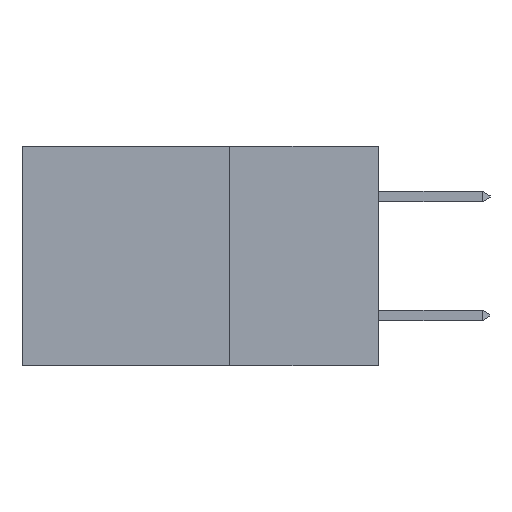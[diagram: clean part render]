
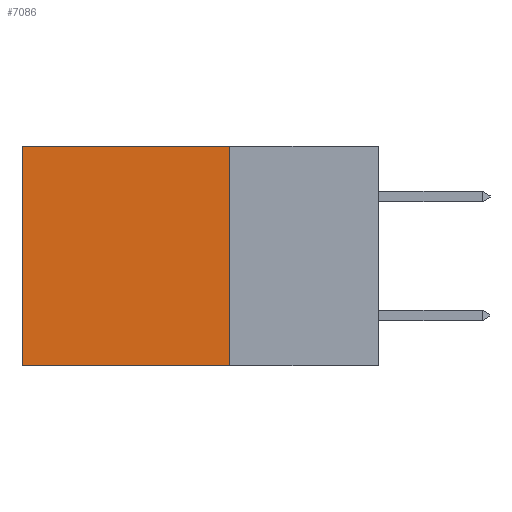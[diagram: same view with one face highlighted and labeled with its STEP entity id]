
A CAD part, left-side view. The second image highlights one B-rep face of the part: STEP entity #7086.
In plain terms, the highlighted planar face has unit normal (-1, 0, 0).
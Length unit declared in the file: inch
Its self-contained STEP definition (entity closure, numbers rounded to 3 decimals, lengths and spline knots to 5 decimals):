
#74 = CARTESIAN_POINT ( 'NONE',  ( 0.298, 0.6, 0. ) ) ;
#310 = EDGE_LOOP ( 'NONE', ( #7199, #5435, #2996, #6718 ) ) ;
#1851 = CARTESIAN_POINT ( 'NONE',  ( 0.298, 0.6, -0.37 ) ) ;
#2135 = LINE ( 'NONE', #3956, #12154 ) ;
#2180 = AXIS2_PLACEMENT_3D ( 'NONE', #2673, #4735, #11431 ) ;
#2197 = EDGE_CURVE ( 'NONE', #12668, #10796, #11174, .T. ) ;
#2673 = CARTESIAN_POINT ( 'NONE',  ( 0.298, 0.25, 0. ) ) ;
#2812 = CARTESIAN_POINT ( 'NONE',  ( 0.298, 0.25, 0. ) ) ;
#2899 = EDGE_CURVE ( 'NONE', #8520, #3314, #2135, .T. ) ;
#2996 = ORIENTED_EDGE ( 'NONE', *, *, #11598, .F. ) ;
#3002 = CARTESIAN_POINT ( 'NONE',  ( 0.298, 0.25, 0. ) ) ;
#3314 = VERTEX_POINT ( 'NONE', #74 ) ;
#3824 = DIRECTION ( 'NONE',  ( 0., 0., -1. ) ) ;
#3956 = CARTESIAN_POINT ( 'NONE',  ( 0.298, 0.25, 0. ) ) ;
#4020 = VECTOR ( 'NONE', #12395, 39.37008 ) ;
#4735 = DIRECTION ( 'NONE',  ( 1., 0., 0. ) ) ;
#5117 = LINE ( 'NONE', #2812, #10001 ) ;
#5435 = ORIENTED_EDGE ( 'NONE', *, *, #2197, .F. ) ;
#5853 = CARTESIAN_POINT ( 'NONE',  ( 0.298, 0.25, -0.37 ) ) ;
#6718 = ORIENTED_EDGE ( 'NONE', *, *, #2899, .T. ) ;
#7034 = CARTESIAN_POINT ( 'NONE',  ( 0.298, 0.25, -0.37 ) ) ;
#7086 = ADVANCED_FACE ( 'NONE', ( #9249 ), #10544, .F. ) ;
#7199 = ORIENTED_EDGE ( 'NONE', *, *, #8305, .T. ) ;
#8305 = EDGE_CURVE ( 'NONE', #3314, #10796, #11991, .T. ) ;
#8520 = VERTEX_POINT ( 'NONE', #3002 ) ;
#8833 = VECTOR ( 'NONE', #12445, 39.37008 ) ;
#9249 = FACE_OUTER_BOUND ( 'NONE', #310, .T. ) ;
#10001 = VECTOR ( 'NONE', #3824, 39.37008 ) ;
#10341 = DIRECTION ( 'NONE',  ( 0., 1., 0. ) ) ;
#10544 = PLANE ( 'NONE',  #2180 ) ;
#10796 = VERTEX_POINT ( 'NONE', #1851 ) ;
#11174 = LINE ( 'NONE', #5853, #8833 ) ;
#11431 = DIRECTION ( 'NONE',  ( 0., 0., -1. ) ) ;
#11495 = CARTESIAN_POINT ( 'NONE',  ( 0.298, 0.6, 0. ) ) ;
#11598 = EDGE_CURVE ( 'NONE', #8520, #12668, #5117, .T. ) ;
#11991 = LINE ( 'NONE', #11495, #4020 ) ;
#12154 = VECTOR ( 'NONE', #10341, 39.37008 ) ;
#12395 = DIRECTION ( 'NONE',  ( 0., 0., -1. ) ) ;
#12445 = DIRECTION ( 'NONE',  ( 0., 1., 0. ) ) ;
#12668 = VERTEX_POINT ( 'NONE', #7034 ) ;
